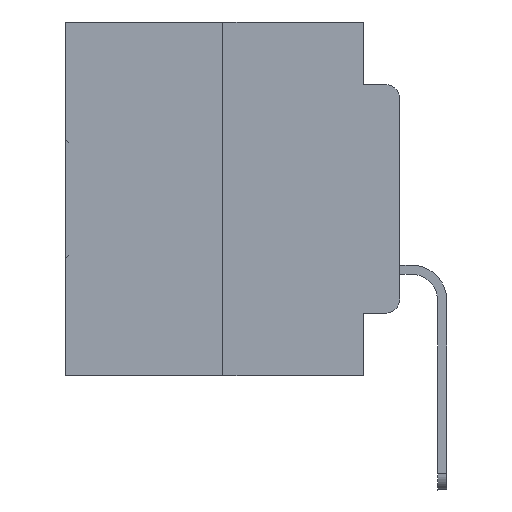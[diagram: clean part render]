
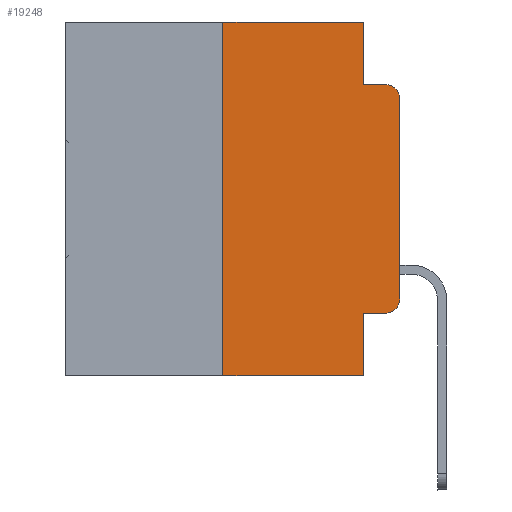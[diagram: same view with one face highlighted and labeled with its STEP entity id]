
A CAD part, left-side view. The second image highlights one B-rep face of the part: STEP entity #19248.
In plain terms, the highlighted planar face has unit normal (-1, 0, 0).
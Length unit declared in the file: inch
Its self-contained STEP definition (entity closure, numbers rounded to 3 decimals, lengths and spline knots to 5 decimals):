
#194 = DIRECTION ( 'NONE',  ( 0., -1., 0. ) ) ;
#245 = DIRECTION ( 'NONE',  ( 0., 0., -1. ) ) ;
#424 = LINE ( 'NONE', #3864, #9795 ) ;
#436 = LINE ( 'NONE', #10113, #24367 ) ;
#473 = CARTESIAN_POINT ( 'NONE',  ( 0., 0.051, 0. ) ) ;
#952 = EDGE_CURVE ( 'NONE', #21036, #16046, #4820, .T. ) ;
#961 = CARTESIAN_POINT ( 'NONE',  ( 0., 0.02, -0.1085 ) ) ;
#1728 = CARTESIAN_POINT ( 'NONE',  ( 0., 0.02, -0.4115 ) ) ;
#1892 = ORIENTED_EDGE ( 'NONE', *, *, #29366, .F. ) ;
#2329 = CARTESIAN_POINT ( 'NONE',  ( 0., 0.051, 0. ) ) ;
#2494 = LINE ( 'NONE', #21172, #5474 ) ;
#2864 = ORIENTED_EDGE ( 'NONE', *, *, #3739, .F. ) ;
#3241 = CARTESIAN_POINT ( 'NONE',  ( 0., 0.051, -0.5 ) ) ;
#3734 = AXIS2_PLACEMENT_3D ( 'NONE', #961, #14619, #12474 ) ;
#3739 = EDGE_CURVE ( 'NONE', #29156, #6365, #2494, .T. ) ;
#3752 = DIRECTION ( 'NONE',  ( 0., 0., -1. ) ) ;
#3864 = CARTESIAN_POINT ( 'NONE',  ( 0., 0., 0. ) ) ;
#3904 = PLANE ( 'NONE',  #8284 ) ;
#4045 = LINE ( 'NONE', #18142, #23309 ) ;
#4820 = LINE ( 'NONE', #9761, #11924 ) ;
#5088 = EDGE_CURVE ( 'NONE', #26887, #16909, #9137, .T. ) ;
#5439 = VECTOR ( 'NONE', #13421, 39.37008 ) ;
#5474 = VECTOR ( 'NONE', #194, 39.37008 ) ;
#5478 = CARTESIAN_POINT ( 'NONE',  ( 0., 0.02, -0.0885 ) ) ;
#6080 = EDGE_CURVE ( 'NONE', #6691, #26887, #424, .T. ) ;
#6365 = VERTEX_POINT ( 'NONE', #473 ) ;
#6691 = VERTEX_POINT ( 'NONE', #9204 ) ;
#7883 = ORIENTED_EDGE ( 'NONE', *, *, #6080, .T. ) ;
#8284 = AXIS2_PLACEMENT_3D ( 'NONE', #11436, #22586, #3752 ) ;
#8867 = ORIENTED_EDGE ( 'NONE', *, *, #5088, .T. ) ;
#9137 = CIRCLE ( 'NONE', #3734, 0.02 ) ;
#9204 = CARTESIAN_POINT ( 'NONE',  ( 0., 0., -0.3915 ) ) ;
#9667 = ORIENTED_EDGE ( 'NONE', *, *, #21999, .F. ) ;
#9761 = CARTESIAN_POINT ( 'NONE',  ( 0., 0.473, -0.5 ) ) ;
#9795 = VECTOR ( 'NONE', #13544, 39.37008 ) ;
#10113 = CARTESIAN_POINT ( 'NONE',  ( 0., 0.051, -0.4115 ) ) ;
#10429 = LINE ( 'NONE', #24033, #10681 ) ;
#10681 = VECTOR ( 'NONE', #13034, 39.37008 ) ;
#10959 = CARTESIAN_POINT ( 'NONE',  ( 0., 0.25, -0.5 ) ) ;
#11169 = EDGE_CURVE ( 'NONE', #21036, #29156, #4045, .T. ) ;
#11259 = LINE ( 'NONE', #2329, #5439 ) ;
#11436 = CARTESIAN_POINT ( 'NONE',  ( 0., 0.473, 0. ) ) ;
#11924 = VECTOR ( 'NONE', #12208, 39.37008 ) ;
#11999 = ORIENTED_EDGE ( 'NONE', *, *, #11169, .F. ) ;
#12097 = DIRECTION ( 'NONE',  ( -1., 0., 0. ) ) ;
#12208 = DIRECTION ( 'NONE',  ( 0., -1., 0. ) ) ;
#12474 = DIRECTION ( 'NONE',  ( 0., 0., -1. ) ) ;
#13034 = DIRECTION ( 'NONE',  ( 0., -1., 0. ) ) ;
#13421 = DIRECTION ( 'NONE',  ( 0., 0., -1. ) ) ;
#13544 = DIRECTION ( 'NONE',  ( 0., 0., 1. ) ) ;
#13777 = LINE ( 'NONE', #20636, #18055 ) ;
#13873 = DIRECTION ( 'NONE',  ( 0., 0., 1. ) ) ;
#14588 = CARTESIAN_POINT ( 'NONE',  ( 0., 0., -0.1085 ) ) ;
#14619 = DIRECTION ( 'NONE',  ( -1., 0., 0. ) ) ;
#14998 = DIRECTION ( 'NONE',  ( 0., 0., -1. ) ) ;
#15048 = CIRCLE ( 'NONE', #19441, 0.02 ) ;
#16046 = VERTEX_POINT ( 'NONE', #3241 ) ;
#16149 = ORIENTED_EDGE ( 'NONE', *, *, #21660, .T. ) ;
#16419 = EDGE_CURVE ( 'NONE', #26024, #16909, #10429, .T. ) ;
#16685 = CARTESIAN_POINT ( 'NONE',  ( 0., 0.02, -0.3915 ) ) ;
#16909 = VERTEX_POINT ( 'NONE', #5478 ) ;
#17290 = EDGE_LOOP ( 'NONE', ( #7883, #8867, #19928, #9667, #2864, #11999, #24078, #1892, #16149, #21845 ) ) ;
#18055 = VECTOR ( 'NONE', #245, 39.37008 ) ;
#18142 = CARTESIAN_POINT ( 'NONE',  ( 0., 0.25, 0. ) ) ;
#19248 = ADVANCED_FACE ( 'NONE', ( #20587 ), #3904, .F. ) ;
#19441 = AXIS2_PLACEMENT_3D ( 'NONE', #16685, #12097, #14998 ) ;
#19928 = ORIENTED_EDGE ( 'NONE', *, *, #16419, .F. ) ;
#20380 = EDGE_CURVE ( 'NONE', #29451, #6691, #15048, .T. ) ;
#20587 = FACE_OUTER_BOUND ( 'NONE', #17290, .T. ) ;
#20636 = CARTESIAN_POINT ( 'NONE',  ( 0., 0.051, 0. ) ) ;
#21036 = VERTEX_POINT ( 'NONE', #10959 ) ;
#21172 = CARTESIAN_POINT ( 'NONE',  ( 0., 0.473, 0. ) ) ;
#21660 = EDGE_CURVE ( 'NONE', #22618, #29451, #436, .T. ) ;
#21845 = ORIENTED_EDGE ( 'NONE', *, *, #20380, .T. ) ;
#21999 = EDGE_CURVE ( 'NONE', #6365, #26024, #13777, .T. ) ;
#22586 = DIRECTION ( 'NONE',  ( 1., 0., 0. ) ) ;
#22618 = VERTEX_POINT ( 'NONE', #28488 ) ;
#23045 = CARTESIAN_POINT ( 'NONE',  ( 0., 0.25, 0. ) ) ;
#23309 = VECTOR ( 'NONE', #13873, 39.37008 ) ;
#24033 = CARTESIAN_POINT ( 'NONE',  ( 0., 0.051, -0.0885 ) ) ;
#24078 = ORIENTED_EDGE ( 'NONE', *, *, #952, .T. ) ;
#24367 = VECTOR ( 'NONE', #26285, 39.37008 ) ;
#26024 = VERTEX_POINT ( 'NONE', #28758 ) ;
#26285 = DIRECTION ( 'NONE',  ( 0., -1., 0. ) ) ;
#26887 = VERTEX_POINT ( 'NONE', #14588 ) ;
#28488 = CARTESIAN_POINT ( 'NONE',  ( 0., 0.051, -0.4115 ) ) ;
#28758 = CARTESIAN_POINT ( 'NONE',  ( 0., 0.051, -0.0885 ) ) ;
#29156 = VERTEX_POINT ( 'NONE', #23045 ) ;
#29366 = EDGE_CURVE ( 'NONE', #22618, #16046, #11259, .T. ) ;
#29451 = VERTEX_POINT ( 'NONE', #1728 ) ;
